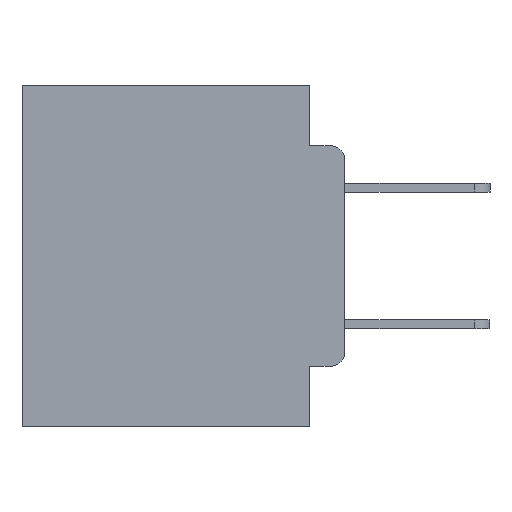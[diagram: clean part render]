
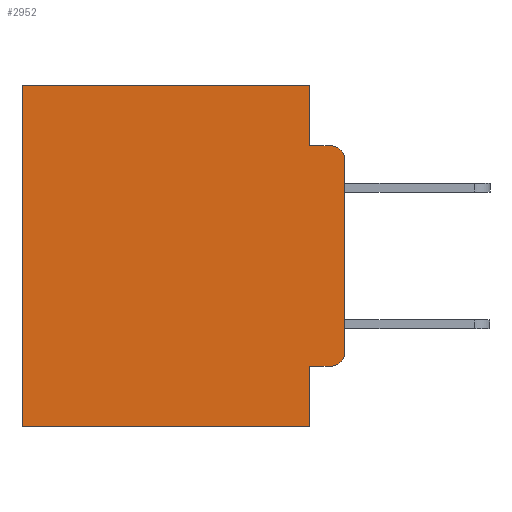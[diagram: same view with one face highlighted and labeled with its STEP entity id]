
A CAD part, left-side view. The second image highlights one B-rep face of the part: STEP entity #2952.
In plain terms, the highlighted planar face has unit normal (-1, 0, 0).
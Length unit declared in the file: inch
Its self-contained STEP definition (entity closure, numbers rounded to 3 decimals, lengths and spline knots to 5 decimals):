
#595 = VERTEX_POINT ( 'NONE', #4206 ) ;
#870 = CARTESIAN_POINT ( 'NONE',  ( 0.298, 0.051, -0.4115 ) ) ;
#1024 = CARTESIAN_POINT ( 'NONE',  ( 0.298, 0.473, 0. ) ) ;
#1169 = LINE ( 'NONE', #23379, #22183 ) ;
#1174 = CARTESIAN_POINT ( 'NONE',  ( 0.298, 0.02, -0.1085 ) ) ;
#1555 = EDGE_CURVE ( 'NONE', #22677, #10801, #13534, .T. ) ;
#2277 = CARTESIAN_POINT ( 'NONE',  ( 0.298, 0., -0.1085 ) ) ;
#2886 = PLANE ( 'NONE',  #21617 ) ;
#2952 = ADVANCED_FACE ( 'NONE', ( #24576 ), #2886, .F. ) ;
#3093 = EDGE_CURVE ( 'NONE', #3336, #10801, #26969, .T. ) ;
#3336 = VERTEX_POINT ( 'NONE', #2277 ) ;
#3497 = DIRECTION ( 'NONE',  ( 0., 0., -1. ) ) ;
#3543 = CIRCLE ( 'NONE', #12145, 0.02 ) ;
#4206 = CARTESIAN_POINT ( 'NONE',  ( 0.298, 0.051, 0. ) ) ;
#5080 = VECTOR ( 'NONE', #16710, 39.37008 ) ;
#5181 = DIRECTION ( 'NONE',  ( 1., 0., 0. ) ) ;
#5665 = DIRECTION ( 'NONE',  ( 0., 0., -1. ) ) ;
#6430 = VERTEX_POINT ( 'NONE', #11168 ) ;
#7363 = DIRECTION ( 'NONE',  ( 0., 1., 0. ) ) ;
#7618 = EDGE_CURVE ( 'NONE', #3336, #10091, #22716, .T. ) ;
#7823 = ORIENTED_EDGE ( 'NONE', *, *, #1555, .F. ) ;
#7994 = EDGE_CURVE ( 'NONE', #6430, #13310, #17429, .T. ) ;
#8553 = ORIENTED_EDGE ( 'NONE', *, *, #22207, .T. ) ;
#8871 = CARTESIAN_POINT ( 'NONE',  ( 0.298, 0., 0. ) ) ;
#8873 = CARTESIAN_POINT ( 'NONE',  ( 0.298, 0.051, -0.4115 ) ) ;
#10091 = VERTEX_POINT ( 'NONE', #25148 ) ;
#10508 = CARTESIAN_POINT ( 'NONE',  ( 0.298, 0.051, -0.0885 ) ) ;
#10631 = ORIENTED_EDGE ( 'NONE', *, *, #20112, .T. ) ;
#10801 = VERTEX_POINT ( 'NONE', #12206 ) ;
#10941 = DIRECTION ( 'NONE',  ( -1., 0., 0. ) ) ;
#11147 = VECTOR ( 'NONE', #22225, 39.37008 ) ;
#11168 = CARTESIAN_POINT ( 'NONE',  ( 0.298, 0.051, -0.5 ) ) ;
#11258 = DIRECTION ( 'NONE',  ( 0., 0., -1. ) ) ;
#11675 = VERTEX_POINT ( 'NONE', #19157 ) ;
#11795 = ORIENTED_EDGE ( 'NONE', *, *, #23099, .T. ) ;
#12145 = AXIS2_PLACEMENT_3D ( 'NONE', #24243, #10941, #26462 ) ;
#12206 = CARTESIAN_POINT ( 'NONE',  ( 0.298, 0.02, -0.0885 ) ) ;
#12210 = ORIENTED_EDGE ( 'NONE', *, *, #21612, .F. ) ;
#13310 = VERTEX_POINT ( 'NONE', #14131 ) ;
#13373 = VERTEX_POINT ( 'NONE', #870 ) ;
#13452 = ORIENTED_EDGE ( 'NONE', *, *, #7994, .F. ) ;
#13534 = LINE ( 'NONE', #28114, #18023 ) ;
#13855 = ORIENTED_EDGE ( 'NONE', *, *, #3093, .T. ) ;
#13868 = LINE ( 'NONE', #26773, #25676 ) ;
#14131 = CARTESIAN_POINT ( 'NONE',  ( 0.298, 0.473, -0.5 ) ) ;
#14974 = CARTESIAN_POINT ( 'NONE',  ( 0.298, 0., 0. ) ) ;
#15579 = VECTOR ( 'NONE', #20066, 39.37008 ) ;
#15640 = EDGE_CURVE ( 'NONE', #11675, #10091, #3543, .T. ) ;
#16317 = CARTESIAN_POINT ( 'NONE',  ( 0.298, 0., -0.5 ) ) ;
#16710 = DIRECTION ( 'NONE',  ( 0., 0., -1. ) ) ;
#16848 = DIRECTION ( 'NONE',  ( -1., 0., 0. ) ) ;
#16899 = LINE ( 'NONE', #1024, #5080 ) ;
#17429 = LINE ( 'NONE', #16317, #28517 ) ;
#17983 = EDGE_LOOP ( 'NONE', ( #23495, #13855, #7823, #26365, #8553, #11795, #13452, #12210, #10631, #28761 ) ) ;
#18023 = VECTOR ( 'NONE', #26993, 39.37008 ) ;
#19157 = CARTESIAN_POINT ( 'NONE',  ( 0.298, 0.02, -0.4115 ) ) ;
#19995 = VERTEX_POINT ( 'NONE', #21834 ) ;
#20066 = DIRECTION ( 'NONE',  ( 0., 1., 0. ) ) ;
#20112 = EDGE_CURVE ( 'NONE', #13373, #11675, #23661, .T. ) ;
#20773 = DIRECTION ( 'NONE',  ( 0., 0., -1. ) ) ;
#21509 = LINE ( 'NONE', #8871, #15579 ) ;
#21612 = EDGE_CURVE ( 'NONE', #13373, #6430, #13868, .T. ) ;
#21617 = AXIS2_PLACEMENT_3D ( 'NONE', #27228, #5181, #20773 ) ;
#21834 = CARTESIAN_POINT ( 'NONE',  ( 0.298, 0.473, 0. ) ) ;
#22016 = VECTOR ( 'NONE', #28229, 39.37008 ) ;
#22183 = VECTOR ( 'NONE', #5665, 39.37008 ) ;
#22207 = EDGE_CURVE ( 'NONE', #595, #19995, #21509, .T. ) ;
#22225 = DIRECTION ( 'NONE',  ( 0., -1., 0. ) ) ;
#22677 = VERTEX_POINT ( 'NONE', #10508 ) ;
#22716 = LINE ( 'NONE', #14974, #22016 ) ;
#23099 = EDGE_CURVE ( 'NONE', #19995, #13310, #16899, .T. ) ;
#23379 = CARTESIAN_POINT ( 'NONE',  ( 0.298, 0.051, 0. ) ) ;
#23495 = ORIENTED_EDGE ( 'NONE', *, *, #7618, .F. ) ;
#23661 = LINE ( 'NONE', #8873, #11147 ) ;
#24243 = CARTESIAN_POINT ( 'NONE',  ( 0.298, 0.02, -0.3915 ) ) ;
#24576 = FACE_OUTER_BOUND ( 'NONE', #17983, .T. ) ;
#25148 = CARTESIAN_POINT ( 'NONE',  ( 0.298, 0., -0.3915 ) ) ;
#25676 = VECTOR ( 'NONE', #11258, 39.37008 ) ;
#26365 = ORIENTED_EDGE ( 'NONE', *, *, #28602, .F. ) ;
#26462 = DIRECTION ( 'NONE',  ( 0., 0., -1. ) ) ;
#26773 = CARTESIAN_POINT ( 'NONE',  ( 0.298, 0.051, 0. ) ) ;
#26942 = AXIS2_PLACEMENT_3D ( 'NONE', #1174, #16848, #3497 ) ;
#26969 = CIRCLE ( 'NONE', #26942, 0.02 ) ;
#26993 = DIRECTION ( 'NONE',  ( 0., -1., 0. ) ) ;
#27228 = CARTESIAN_POINT ( 'NONE',  ( 0.298, 0., 0. ) ) ;
#28114 = CARTESIAN_POINT ( 'NONE',  ( 0.298, 0.051, -0.0885 ) ) ;
#28229 = DIRECTION ( 'NONE',  ( 0., 0., -1. ) ) ;
#28517 = VECTOR ( 'NONE', #7363, 39.37008 ) ;
#28602 = EDGE_CURVE ( 'NONE', #595, #22677, #1169, .T. ) ;
#28761 = ORIENTED_EDGE ( 'NONE', *, *, #15640, .T. ) ;
